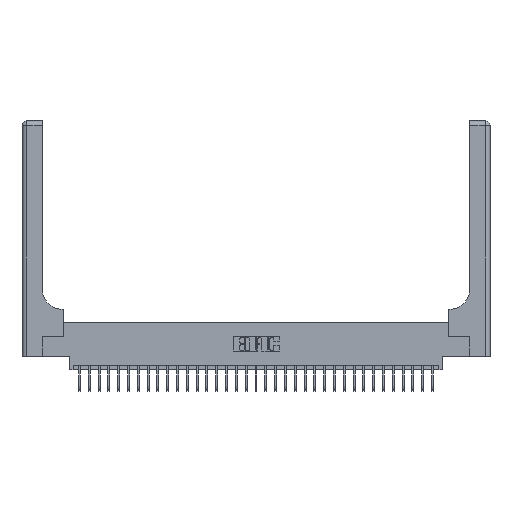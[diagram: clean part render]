
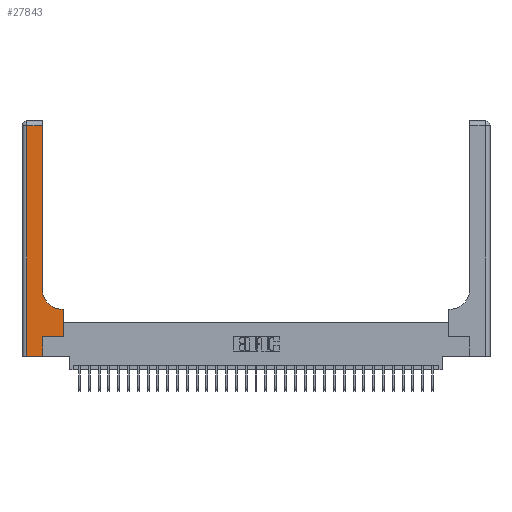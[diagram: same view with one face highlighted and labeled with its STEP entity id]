
A CAD part, top view. The second image highlights one B-rep face of the part: STEP entity #27843.
In plain terms, the highlighted planar face has unit normal (0, 0, 1).
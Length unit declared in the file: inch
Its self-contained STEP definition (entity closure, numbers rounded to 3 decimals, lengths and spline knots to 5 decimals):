
#153 = CARTESIAN_POINT ( 'NONE',  ( 0., 2.94, 0.37 ) ) ;
#205 = EDGE_CURVE ( 'NONE', #10671, #13363, #3878, .T. ) ;
#341 = CARTESIAN_POINT ( 'NONE',  ( 0.26, 3., 0.37 ) ) ;
#2580 = DIRECTION ( 'NONE',  ( 0., 0., -1. ) ) ;
#2868 = VERTEX_POINT ( 'NONE', #22554 ) ;
#3029 = CARTESIAN_POINT ( 'NONE',  ( 0.26, 0.85, 0.37 ) ) ;
#3741 = LINE ( 'NONE', #13952, #26869 ) ;
#3878 = LINE ( 'NONE', #341, #21052 ) ;
#5489 = CARTESIAN_POINT ( 'NONE',  ( 0.265, 0., 0.37 ) ) ;
#6356 = VERTEX_POINT ( 'NONE', #13423 ) ;
#6390 = CARTESIAN_POINT ( 'NONE',  ( 0., 0., 0.37 ) ) ;
#6880 = EDGE_CURVE ( 'NONE', #23804, #10671, #8619, .T. ) ;
#6918 = DIRECTION ( 'NONE',  ( -1., 0., 0. ) ) ;
#6921 = DIRECTION ( 'NONE',  ( 0., 0., -1. ) ) ;
#7290 = CARTESIAN_POINT ( 'NONE',  ( 0.265, 0., 0.37 ) ) ;
#7294 = DIRECTION ( 'NONE',  ( -1., 0., 0. ) ) ;
#8003 = AXIS2_PLACEMENT_3D ( 'NONE', #9273, #2580, #18251 ) ;
#8619 = CIRCLE ( 'NONE', #10080, 0.25 ) ;
#8636 = DIRECTION ( 'NONE',  ( 1., 0., 0. ) ) ;
#8713 = ORIENTED_EDGE ( 'NONE', *, *, #14390, .T. ) ;
#8871 = LINE ( 'NONE', #6390, #20080 ) ;
#8953 = VECTOR ( 'NONE', #20733, 39.37008 ) ;
#9226 = CARTESIAN_POINT ( 'NONE',  ( 0.265, 0.25, 0.37 ) ) ;
#9273 = CARTESIAN_POINT ( 'NONE',  ( 0., 3., 0.37 ) ) ;
#10080 = AXIS2_PLACEMENT_3D ( 'NONE', #20363, #6921, #22627 ) ;
#10540 = VERTEX_POINT ( 'NONE', #9226 ) ;
#10671 = VERTEX_POINT ( 'NONE', #3029 ) ;
#11636 = DIRECTION ( 'NONE',  ( 0., 1., 0. ) ) ;
#11662 = LINE ( 'NONE', #153, #28824 ) ;
#11718 = ORIENTED_EDGE ( 'NONE', *, *, #13023, .T. ) ;
#11747 = EDGE_CURVE ( 'NONE', #6356, #2868, #20283, .T. ) ;
#12246 = ORIENTED_EDGE ( 'NONE', *, *, #17415, .T. ) ;
#12746 = ORIENTED_EDGE ( 'NONE', *, *, #6880, .T. ) ;
#13023 = EDGE_CURVE ( 'NONE', #23750, #23804, #3741, .T. ) ;
#13363 = VERTEX_POINT ( 'NONE', #19527 ) ;
#13423 = CARTESIAN_POINT ( 'NONE',  ( 0.06, 2.94, 0.37 ) ) ;
#13854 = VERTEX_POINT ( 'NONE', #5489 ) ;
#13952 = CARTESIAN_POINT ( 'NONE',  ( 0.26, 0.6, 0.37 ) ) ;
#14390 = EDGE_CURVE ( 'NONE', #10540, #24123, #14726, .T. ) ;
#14398 = DIRECTION ( 'NONE',  ( 0., 1., 0. ) ) ;
#14726 = LINE ( 'NONE', #25561, #25974 ) ;
#16005 = PLANE ( 'NONE',  #8003 ) ;
#17283 = CARTESIAN_POINT ( 'NONE',  ( 0.528, 0.25, 0.37 ) ) ;
#17415 = EDGE_CURVE ( 'NONE', #13854, #10540, #20873, .T. ) ;
#17878 = VECTOR ( 'NONE', #14398, 39.37008 ) ;
#18251 = DIRECTION ( 'NONE',  ( -1., 0., 0. ) ) ;
#18397 = CARTESIAN_POINT ( 'NONE',  ( 0.51, 0.6, 0.37 ) ) ;
#18868 = DIRECTION ( 'NONE',  ( 1., 0., 0. ) ) ;
#18869 = VECTOR ( 'NONE', #19730, 39.37008 ) ;
#18961 = ORIENTED_EDGE ( 'NONE', *, *, #25567, .T. ) ;
#19313 = LINE ( 'NONE', #23420, #17878 ) ;
#19527 = CARTESIAN_POINT ( 'NONE',  ( 0.26, 2.94, 0.37 ) ) ;
#19540 = EDGE_CURVE ( 'NONE', #2868, #13854, #8871, .T. ) ;
#19730 = DIRECTION ( 'NONE',  ( 0., -1., 0. ) ) ;
#19814 = CARTESIAN_POINT ( 'NONE',  ( 0.06, 3., 0.37 ) ) ;
#19971 = EDGE_CURVE ( 'NONE', #24123, #23750, #19313, .T. ) ;
#20080 = VECTOR ( 'NONE', #8636, 39.37008 ) ;
#20283 = LINE ( 'NONE', #19814, #18869 ) ;
#20363 = CARTESIAN_POINT ( 'NONE',  ( 0.51, 0.85, 0.37 ) ) ;
#20733 = DIRECTION ( 'NONE',  ( 0., 1., 0. ) ) ;
#20873 = LINE ( 'NONE', #7290, #8953 ) ;
#21052 = VECTOR ( 'NONE', #11636, 39.37008 ) ;
#22305 = FACE_OUTER_BOUND ( 'NONE', #28776, .T. ) ;
#22554 = CARTESIAN_POINT ( 'NONE',  ( 0.06, 0., 0.37 ) ) ;
#22627 = DIRECTION ( 'NONE',  ( 1., 0., 0. ) ) ;
#23420 = CARTESIAN_POINT ( 'NONE',  ( 0.528, 0.25, 0.37 ) ) ;
#23750 = VERTEX_POINT ( 'NONE', #27232 ) ;
#23804 = VERTEX_POINT ( 'NONE', #18397 ) ;
#24123 = VERTEX_POINT ( 'NONE', #17283 ) ;
#25119 = ORIENTED_EDGE ( 'NONE', *, *, #19971, .T. ) ;
#25561 = CARTESIAN_POINT ( 'NONE',  ( 0.265, 0.25, 0.37 ) ) ;
#25567 = EDGE_CURVE ( 'NONE', #13363, #6356, #11662, .T. ) ;
#25974 = VECTOR ( 'NONE', #18868, 39.37008 ) ;
#26869 = VECTOR ( 'NONE', #7294, 39.37008 ) ;
#27232 = CARTESIAN_POINT ( 'NONE',  ( 0.528, 0.6, 0.37 ) ) ;
#27649 = ORIENTED_EDGE ( 'NONE', *, *, #11747, .T. ) ;
#27843 = ADVANCED_FACE ( 'NONE', ( #22305 ), #16005, .F. ) ;
#28264 = ORIENTED_EDGE ( 'NONE', *, *, #205, .T. ) ;
#28445 = ORIENTED_EDGE ( 'NONE', *, *, #19540, .T. ) ;
#28776 = EDGE_LOOP ( 'NONE', ( #28264, #18961, #27649, #28445, #12246, #8713, #25119, #11718, #12746 ) ) ;
#28824 = VECTOR ( 'NONE', #6918, 39.37008 ) ;
